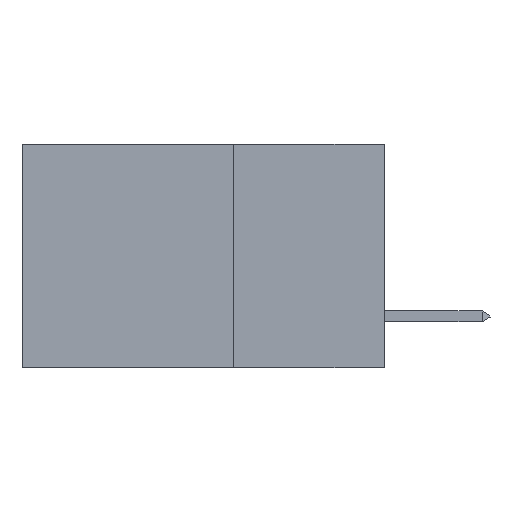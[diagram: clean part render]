
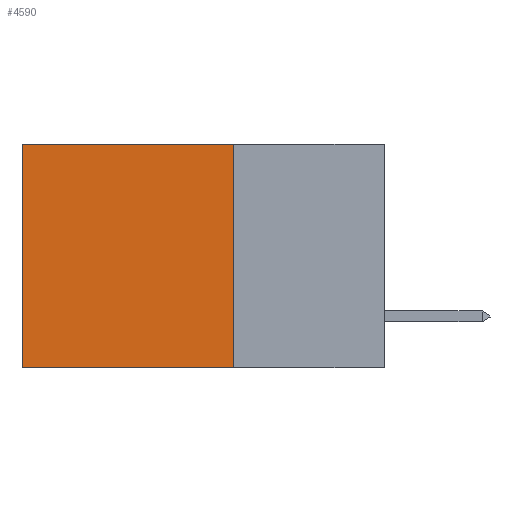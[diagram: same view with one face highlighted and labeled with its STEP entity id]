
A CAD part, left-side view. The second image highlights one B-rep face of the part: STEP entity #4590.
In plain terms, the highlighted planar face has unit normal (-1, 0, 0).
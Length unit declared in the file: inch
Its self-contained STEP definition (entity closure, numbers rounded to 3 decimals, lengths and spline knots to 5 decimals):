
#153 = VERTEX_POINT ( 'NONE', #31025 ) ;
#651 = LINE ( 'NONE', #15557, #36324 ) ;
#1213 = DIRECTION ( 'NONE',  ( 1., 0., 0. ) ) ;
#1811 = CARTESIAN_POINT ( 'NONE',  ( 0.2875, 0.6, 0. ) ) ;
#1946 = LINE ( 'NONE', #2902, #14898 ) ;
#2902 = CARTESIAN_POINT ( 'NONE',  ( 0.2875, 0.25, 0. ) ) ;
#4156 = ORIENTED_EDGE ( 'NONE', *, *, #14098, .F. ) ;
#4590 = ADVANCED_FACE ( 'NONE', ( #13337 ), #22081, .F. ) ;
#4900 = LINE ( 'NONE', #44091, #40543 ) ;
#5441 = CARTESIAN_POINT ( 'NONE',  ( 0.2875, 0.25, 0. ) ) ;
#7549 = EDGE_CURVE ( 'NONE', #35485, #153, #40094, .T. ) ;
#7996 = CARTESIAN_POINT ( 'NONE',  ( 0.2875, 0.25, 0. ) ) ;
#11478 = VERTEX_POINT ( 'NONE', #5441 ) ;
#13337 = FACE_OUTER_BOUND ( 'NONE', #19791, .T. ) ;
#14098 = EDGE_CURVE ( 'NONE', #11478, #35485, #4900, .T. ) ;
#14468 = ORIENTED_EDGE ( 'NONE', *, *, #16949, .T. ) ;
#14898 = VECTOR ( 'NONE', #39230, 39.37008 ) ;
#15557 = CARTESIAN_POINT ( 'NONE',  ( 0.2875, 0.6, 0. ) ) ;
#16949 = EDGE_CURVE ( 'NONE', #11478, #23856, #1946, .T. ) ;
#17447 = VECTOR ( 'NONE', #25608, 39.37008 ) ;
#19791 = EDGE_LOOP ( 'NONE', ( #23049, #21548, #4156, #14468 ) ) ;
#21548 = ORIENTED_EDGE ( 'NONE', *, *, #7549, .F. ) ;
#22081 = PLANE ( 'NONE',  #28852 ) ;
#23049 = ORIENTED_EDGE ( 'NONE', *, *, #34021, .T. ) ;
#23856 = VERTEX_POINT ( 'NONE', #1811 ) ;
#24629 = CARTESIAN_POINT ( 'NONE',  ( 0.2875, 0.25, -0.37 ) ) ;
#25608 = DIRECTION ( 'NONE',  ( 0., 1., 0. ) ) ;
#28852 = AXIS2_PLACEMENT_3D ( 'NONE', #7996, #1213, #35635 ) ;
#29223 = CARTESIAN_POINT ( 'NONE',  ( 0.2875, 0.25, -0.37 ) ) ;
#31025 = CARTESIAN_POINT ( 'NONE',  ( 0.2875, 0.6, -0.37 ) ) ;
#34021 = EDGE_CURVE ( 'NONE', #23856, #153, #651, .T. ) ;
#35485 = VERTEX_POINT ( 'NONE', #24629 ) ;
#35635 = DIRECTION ( 'NONE',  ( 0., 0., -1. ) ) ;
#36324 = VECTOR ( 'NONE', #43894, 39.37008 ) ;
#38787 = DIRECTION ( 'NONE',  ( 0., 0., -1. ) ) ;
#39230 = DIRECTION ( 'NONE',  ( 0., 1., 0. ) ) ;
#40094 = LINE ( 'NONE', #29223, #17447 ) ;
#40543 = VECTOR ( 'NONE', #38787, 39.37008 ) ;
#43894 = DIRECTION ( 'NONE',  ( 0., 0., -1. ) ) ;
#44091 = CARTESIAN_POINT ( 'NONE',  ( 0.2875, 0.25, 0. ) ) ;
